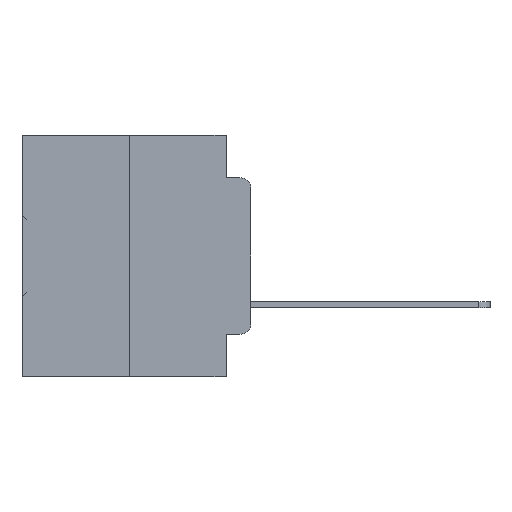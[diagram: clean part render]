
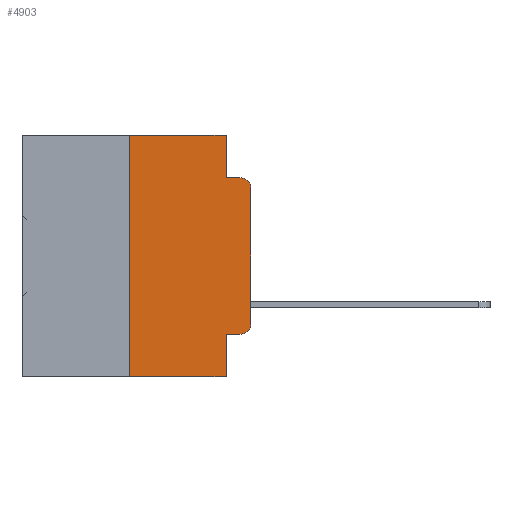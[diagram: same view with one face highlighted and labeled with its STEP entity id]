
A CAD part, left-side view. The second image highlights one B-rep face of the part: STEP entity #4903.
In plain terms, the highlighted planar face has unit normal (-1, 0, 0).
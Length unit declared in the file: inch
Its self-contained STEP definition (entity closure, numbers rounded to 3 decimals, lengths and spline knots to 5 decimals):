
#593 = DIRECTION ( 'NONE',  ( 0., 0., -1. ) ) ;
#683 = VERTEX_POINT ( 'NONE', #30469 ) ;
#1138 = ORIENTED_EDGE ( 'NONE', *, *, #24575, .T. ) ;
#1337 = VERTEX_POINT ( 'NONE', #13470 ) ;
#2468 = VECTOR ( 'NONE', #15823, 39.37008 ) ;
#3062 = DIRECTION ( 'NONE',  ( 0., 0., 1. ) ) ;
#4166 = EDGE_CURVE ( 'NONE', #23521, #1337, #37258, .T. ) ;
#4698 = CARTESIAN_POINT ( 'NONE',  ( 0., 0.051, 0. ) ) ;
#4903 = ADVANCED_FACE ( 'NONE', ( #4999 ), #9490, .F. ) ;
#4999 = FACE_OUTER_BOUND ( 'NONE', #21373, .T. ) ;
#6344 = CARTESIAN_POINT ( 'NONE',  ( 0., 0.051, -0.4115 ) ) ;
#6751 = ORIENTED_EDGE ( 'NONE', *, *, #4166, .F. ) ;
#6978 = VECTOR ( 'NONE', #35486, 39.37008 ) ;
#7497 = VECTOR ( 'NONE', #36869, 39.37008 ) ;
#7612 = CARTESIAN_POINT ( 'NONE',  ( 0., 0.02, -0.4115 ) ) ;
#8124 = CARTESIAN_POINT ( 'NONE',  ( 0., 0.051, -0.4115 ) ) ;
#8328 = VECTOR ( 'NONE', #37468, 39.37008 ) ;
#8367 = VERTEX_POINT ( 'NONE', #7612 ) ;
#8745 = VECTOR ( 'NONE', #28313, 39.37008 ) ;
#9341 = CARTESIAN_POINT ( 'NONE',  ( 0., 0.051, -0.5 ) ) ;
#9434 = CARTESIAN_POINT ( 'NONE',  ( 0., 0.473, -0.5 ) ) ;
#9490 = PLANE ( 'NONE',  #35949 ) ;
#9697 = LINE ( 'NONE', #34036, #8745 ) ;
#10292 = LINE ( 'NONE', #19718, #7497 ) ;
#10319 = CARTESIAN_POINT ( 'NONE',  ( 0., 0.02, -0.0885 ) ) ;
#11537 = CARTESIAN_POINT ( 'NONE',  ( 0., 0.25, 0. ) ) ;
#11838 = ORIENTED_EDGE ( 'NONE', *, *, #14072, .F. ) ;
#13265 = LINE ( 'NONE', #4698, #27784 ) ;
#13470 = CARTESIAN_POINT ( 'NONE',  ( 0., 0.25, 0. ) ) ;
#13609 = ORIENTED_EDGE ( 'NONE', *, *, #35349, .T. ) ;
#13655 = ORIENTED_EDGE ( 'NONE', *, *, #29528, .F. ) ;
#14072 = EDGE_CURVE ( 'NONE', #32551, #19979, #13265, .T. ) ;
#14088 = ORIENTED_EDGE ( 'NONE', *, *, #29599, .T. ) ;
#14129 = ORIENTED_EDGE ( 'NONE', *, *, #34126, .F. ) ;
#14348 = CARTESIAN_POINT ( 'NONE',  ( 0., 0.051, -0.0885 ) ) ;
#15823 = DIRECTION ( 'NONE',  ( 0., -1., 0. ) ) ;
#16217 = VERTEX_POINT ( 'NONE', #8124 ) ;
#16277 = CARTESIAN_POINT ( 'NONE',  ( 0., 0.02, -0.3915 ) ) ;
#16629 = LINE ( 'NONE', #9434, #6978 ) ;
#17000 = VECTOR ( 'NONE', #35382, 39.37008 ) ;
#17069 = CARTESIAN_POINT ( 'NONE',  ( 0., 0.02, -0.1085 ) ) ;
#17789 = CARTESIAN_POINT ( 'NONE',  ( 0., 0., 0. ) ) ;
#18021 = EDGE_CURVE ( 'NONE', #19979, #28891, #19094, .T. ) ;
#18340 = DIRECTION ( 'NONE',  ( 1., 0., 0. ) ) ;
#18731 = EDGE_CURVE ( 'NONE', #8367, #19052, #24508, .T. ) ;
#19052 = VERTEX_POINT ( 'NONE', #27119 ) ;
#19094 = LINE ( 'NONE', #33075, #2468 ) ;
#19201 = DIRECTION ( 'NONE',  ( 0., 0., -1. ) ) ;
#19718 = CARTESIAN_POINT ( 'NONE',  ( 0., 0.051, 0. ) ) ;
#19976 = DIRECTION ( 'NONE',  ( 0., 0., -1. ) ) ;
#19979 = VERTEX_POINT ( 'NONE', #14348 ) ;
#21373 = EDGE_LOOP ( 'NONE', ( #13609, #14088, #26387, #11838, #13655, #6751, #24166, #14129, #1138, #24626 ) ) ;
#23401 = CIRCLE ( 'NONE', #37244, 0.02 ) ;
#23521 = VERTEX_POINT ( 'NONE', #27025 ) ;
#24166 = ORIENTED_EDGE ( 'NONE', *, *, #28730, .T. ) ;
#24408 = CARTESIAN_POINT ( 'NONE',  ( 0., 0.051, 0. ) ) ;
#24508 = CIRCLE ( 'NONE', #26731, 0.02 ) ;
#24575 = EDGE_CURVE ( 'NONE', #16217, #8367, #24729, .T. ) ;
#24626 = ORIENTED_EDGE ( 'NONE', *, *, #18731, .T. ) ;
#24729 = LINE ( 'NONE', #6344, #17000 ) ;
#25202 = DIRECTION ( 'NONE',  ( 0., 0., -1. ) ) ;
#26387 = ORIENTED_EDGE ( 'NONE', *, *, #18021, .F. ) ;
#26731 = AXIS2_PLACEMENT_3D ( 'NONE', #16277, #36399, #19201 ) ;
#27025 = CARTESIAN_POINT ( 'NONE',  ( 0., 0.25, -0.5 ) ) ;
#27119 = CARTESIAN_POINT ( 'NONE',  ( 0., 0., -0.3915 ) ) ;
#27784 = VECTOR ( 'NONE', #25202, 39.37008 ) ;
#28313 = DIRECTION ( 'NONE',  ( 0., -1., 0. ) ) ;
#28730 = EDGE_CURVE ( 'NONE', #23521, #34352, #16629, .T. ) ;
#28891 = VERTEX_POINT ( 'NONE', #10319 ) ;
#29528 = EDGE_CURVE ( 'NONE', #1337, #32551, #9697, .T. ) ;
#29599 = EDGE_CURVE ( 'NONE', #683, #28891, #23401, .T. ) ;
#30108 = VECTOR ( 'NONE', #3062, 39.37008 ) ;
#30469 = CARTESIAN_POINT ( 'NONE',  ( 0., 0., -0.1085 ) ) ;
#32551 = VERTEX_POINT ( 'NONE', #24408 ) ;
#32656 = CARTESIAN_POINT ( 'NONE',  ( 0., 0.473, 0. ) ) ;
#33075 = CARTESIAN_POINT ( 'NONE',  ( 0., 0.051, -0.0885 ) ) ;
#34036 = CARTESIAN_POINT ( 'NONE',  ( 0., 0.473, 0. ) ) ;
#34126 = EDGE_CURVE ( 'NONE', #16217, #34352, #10292, .T. ) ;
#34352 = VERTEX_POINT ( 'NONE', #9341 ) ;
#35349 = EDGE_CURVE ( 'NONE', #19052, #683, #37692, .T. ) ;
#35382 = DIRECTION ( 'NONE',  ( 0., -1., 0. ) ) ;
#35486 = DIRECTION ( 'NONE',  ( 0., -1., 0. ) ) ;
#35949 = AXIS2_PLACEMENT_3D ( 'NONE', #32656, #18340, #593 ) ;
#36399 = DIRECTION ( 'NONE',  ( -1., 0., 0. ) ) ;
#36869 = DIRECTION ( 'NONE',  ( 0., 0., -1. ) ) ;
#37144 = DIRECTION ( 'NONE',  ( -1., 0., 0. ) ) ;
#37244 = AXIS2_PLACEMENT_3D ( 'NONE', #17069, #37144, #19976 ) ;
#37258 = LINE ( 'NONE', #11537, #8328 ) ;
#37468 = DIRECTION ( 'NONE',  ( 0., 0., 1. ) ) ;
#37692 = LINE ( 'NONE', #17789, #30108 ) ;
